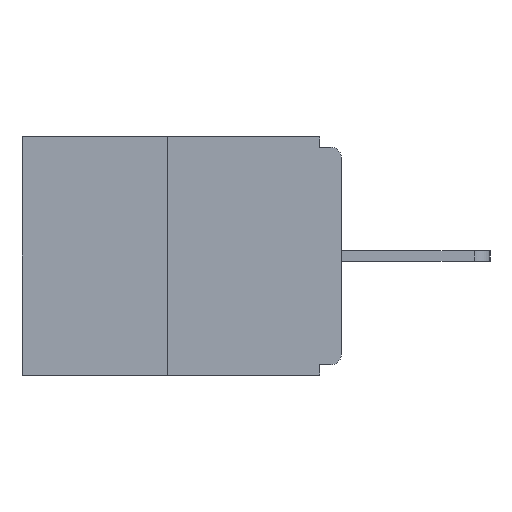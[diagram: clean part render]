
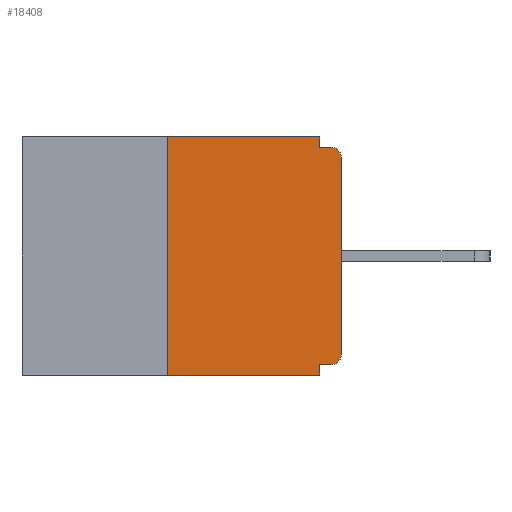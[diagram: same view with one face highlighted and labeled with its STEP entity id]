
A CAD part, left-side view. The second image highlights one B-rep face of the part: STEP entity #18408.
In plain terms, the highlighted planar face has unit normal (-1, 0, 0).
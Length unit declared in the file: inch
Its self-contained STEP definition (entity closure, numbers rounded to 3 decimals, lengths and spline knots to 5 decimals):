
#48 = EDGE_CURVE ( 'NONE', #17685, #20220, #11120, .T. ) ;
#107 = VECTOR ( 'NONE', #11443, 39.37008 ) ;
#460 = VECTOR ( 'NONE', #13970, 39.37008 ) ;
#466 = CIRCLE ( 'NONE', #11615, 0.015 ) ;
#530 = CARTESIAN_POINT ( 'NONE',  ( 0., 0.031, -0.328 ) ) ;
#707 = EDGE_CURVE ( 'NONE', #19406, #2065, #7167, .T. ) ;
#969 = PLANE ( 'NONE',  #10026 ) ;
#1457 = CARTESIAN_POINT ( 'NONE',  ( 0., 0., 0. ) ) ;
#1514 = LINE ( 'NONE', #2793, #18354 ) ;
#1875 = VERTEX_POINT ( 'NONE', #530 ) ;
#1896 = DIRECTION ( 'NONE',  ( 0., -1., 0. ) ) ;
#1928 = EDGE_LOOP ( 'NONE', ( #19823, #15880, #18351, #12919, #2886, #20149, #5129, #20019, #1965, #8562 ) ) ;
#1965 = ORIENTED_EDGE ( 'NONE', *, *, #707, .F. ) ;
#2008 = DIRECTION ( 'NONE',  ( 0., -1., 0. ) ) ;
#2065 = VERTEX_POINT ( 'NONE', #3035 ) ;
#2367 = DIRECTION ( 'NONE',  ( 0., 0., -1. ) ) ;
#2622 = VERTEX_POINT ( 'NONE', #6482 ) ;
#2694 = DIRECTION ( 'NONE',  ( 0., 0., -1. ) ) ;
#2793 = CARTESIAN_POINT ( 'NONE',  ( 0., 0.031, -0.343 ) ) ;
#2886 = ORIENTED_EDGE ( 'NONE', *, *, #14920, .F. ) ;
#3035 = CARTESIAN_POINT ( 'NONE',  ( 0., 0.015, -0.015 ) ) ;
#3460 = CARTESIAN_POINT ( 'NONE',  ( 0., 0., -0.015 ) ) ;
#3565 = CARTESIAN_POINT ( 'NONE',  ( 0., 0.015, -0.03 ) ) ;
#3793 = DIRECTION ( 'NONE',  ( 0., 0., 1. ) ) ;
#3826 = EDGE_CURVE ( 'NONE', #16826, #17685, #466, .T. ) ;
#3848 = LINE ( 'NONE', #8656, #20541 ) ;
#4012 = CARTESIAN_POINT ( 'NONE',  ( 0., 0.031, 0. ) ) ;
#4583 = LINE ( 'NONE', #19354, #107 ) ;
#4845 = VECTOR ( 'NONE', #10363, 39.37008 ) ;
#5121 = VERTEX_POINT ( 'NONE', #4012 ) ;
#5129 = ORIENTED_EDGE ( 'NONE', *, *, #48, .T. ) ;
#5171 = EDGE_CURVE ( 'NONE', #10432, #6373, #8282, .T. ) ;
#5257 = DIRECTION ( 'NONE',  ( 0., 0., -1. ) ) ;
#5679 = CARTESIAN_POINT ( 'NONE',  ( 0., 0., -0.313 ) ) ;
#5850 = DIRECTION ( 'NONE',  ( 0., 0., 1. ) ) ;
#6028 = CARTESIAN_POINT ( 'NONE',  ( 0., 0.46, 0. ) ) ;
#6373 = VERTEX_POINT ( 'NONE', #8607 ) ;
#6482 = CARTESIAN_POINT ( 'NONE',  ( 0., 0.031, -0.343 ) ) ;
#7167 = LINE ( 'NONE', #3460, #10984 ) ;
#7973 = CARTESIAN_POINT ( 'NONE',  ( 0., 0.015, -0.328 ) ) ;
#8068 = FACE_OUTER_BOUND ( 'NONE', #1928, .T. ) ;
#8282 = LINE ( 'NONE', #15698, #21000 ) ;
#8562 = ORIENTED_EDGE ( 'NONE', *, *, #11214, .F. ) ;
#8607 = CARTESIAN_POINT ( 'NONE',  ( 0., 0.25, 0. ) ) ;
#8656 = CARTESIAN_POINT ( 'NONE',  ( 0., 0.46, -0.343 ) ) ;
#9252 = LINE ( 'NONE', #16672, #4845 ) ;
#9366 = LINE ( 'NONE', #12373, #460 ) ;
#9502 = DIRECTION ( 'NONE',  ( 0., 0., -1. ) ) ;
#10026 = AXIS2_PLACEMENT_3D ( 'NONE', #6028, #12573, #2694 ) ;
#10169 = CARTESIAN_POINT ( 'NONE',  ( 0., 0.031, -0.015 ) ) ;
#10363 = DIRECTION ( 'NONE',  ( 0., -1., 0. ) ) ;
#10432 = VERTEX_POINT ( 'NONE', #11080 ) ;
#10984 = VECTOR ( 'NONE', #1896, 39.37008 ) ;
#11080 = CARTESIAN_POINT ( 'NONE',  ( 0., 0.25, -0.343 ) ) ;
#11120 = LINE ( 'NONE', #1457, #19079 ) ;
#11214 = EDGE_CURVE ( 'NONE', #5121, #19406, #9366, .T. ) ;
#11443 = DIRECTION ( 'NONE',  ( 0., 1., 0. ) ) ;
#11615 = AXIS2_PLACEMENT_3D ( 'NONE', #15962, #15881, #2367 ) ;
#12172 = EDGE_CURVE ( 'NONE', #10432, #2622, #3848, .T. ) ;
#12373 = CARTESIAN_POINT ( 'NONE',  ( 0., 0.031, 0. ) ) ;
#12573 = DIRECTION ( 'NONE',  ( 1., 0., 0. ) ) ;
#12919 = ORIENTED_EDGE ( 'NONE', *, *, #17875, .F. ) ;
#13970 = DIRECTION ( 'NONE',  ( 0., 0., -1. ) ) ;
#14180 = CIRCLE ( 'NONE', #20633, 0.015 ) ;
#14474 = EDGE_CURVE ( 'NONE', #6373, #5121, #9252, .T. ) ;
#14645 = CARTESIAN_POINT ( 'NONE',  ( 0., 0., -0.03 ) ) ;
#14920 = EDGE_CURVE ( 'NONE', #16826, #1875, #4583, .T. ) ;
#14991 = DIRECTION ( 'NONE',  ( -1., 0., 0. ) ) ;
#15698 = CARTESIAN_POINT ( 'NONE',  ( 0., 0.25, 0. ) ) ;
#15880 = ORIENTED_EDGE ( 'NONE', *, *, #5171, .F. ) ;
#15881 = DIRECTION ( 'NONE',  ( -1., 0., 0. ) ) ;
#15962 = CARTESIAN_POINT ( 'NONE',  ( 0., 0.015, -0.313 ) ) ;
#16672 = CARTESIAN_POINT ( 'NONE',  ( 0., 0.46, 0. ) ) ;
#16826 = VERTEX_POINT ( 'NONE', #7973 ) ;
#17017 = EDGE_CURVE ( 'NONE', #20220, #2065, #14180, .T. ) ;
#17685 = VERTEX_POINT ( 'NONE', #5679 ) ;
#17875 = EDGE_CURVE ( 'NONE', #1875, #2622, #1514, .T. ) ;
#18351 = ORIENTED_EDGE ( 'NONE', *, *, #12172, .T. ) ;
#18354 = VECTOR ( 'NONE', #9502, 39.37008 ) ;
#18408 = ADVANCED_FACE ( 'NONE', ( #8068 ), #969, .F. ) ;
#19079 = VECTOR ( 'NONE', #3793, 39.37008 ) ;
#19354 = CARTESIAN_POINT ( 'NONE',  ( 0., 0., -0.328 ) ) ;
#19406 = VERTEX_POINT ( 'NONE', #10169 ) ;
#19823 = ORIENTED_EDGE ( 'NONE', *, *, #14474, .F. ) ;
#20019 = ORIENTED_EDGE ( 'NONE', *, *, #17017, .T. ) ;
#20149 = ORIENTED_EDGE ( 'NONE', *, *, #3826, .T. ) ;
#20220 = VERTEX_POINT ( 'NONE', #14645 ) ;
#20541 = VECTOR ( 'NONE', #2008, 39.37008 ) ;
#20633 = AXIS2_PLACEMENT_3D ( 'NONE', #3565, #14991, #5257 ) ;
#21000 = VECTOR ( 'NONE', #5850, 39.37008 ) ;
